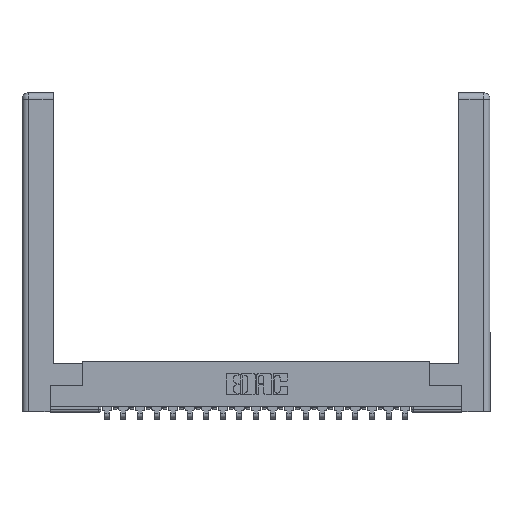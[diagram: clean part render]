
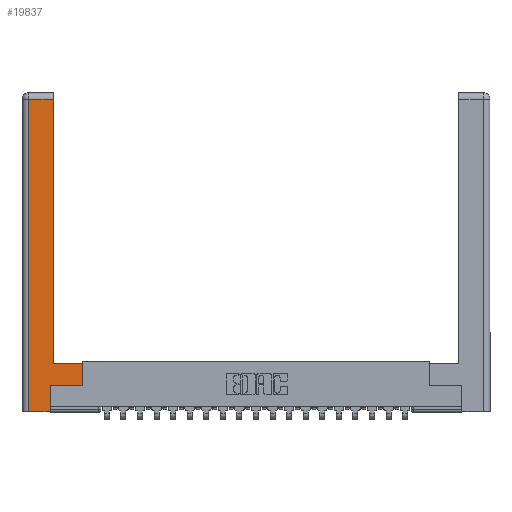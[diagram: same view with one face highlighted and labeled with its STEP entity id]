
A CAD part, top view. The second image highlights one B-rep face of the part: STEP entity #19837.
In plain terms, the highlighted planar face has unit normal (0, 0, 1).
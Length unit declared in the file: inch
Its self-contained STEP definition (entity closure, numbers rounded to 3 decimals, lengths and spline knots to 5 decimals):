
#886 = CARTESIAN_POINT ( 'NONE',  ( 0.565, 0.245, 0. ) ) ;
#1089 = DIRECTION ( 'NONE',  ( -1., 0., 0. ) ) ;
#1253 = ORIENTED_EDGE ( 'NONE', *, *, #11231, .T. ) ;
#1333 = VERTEX_POINT ( 'NONE', #20462 ) ;
#1446 = ORIENTED_EDGE ( 'NONE', *, *, #7583, .T. ) ;
#1805 = VECTOR ( 'NONE', #12024, 39.37008 ) ;
#2521 = FACE_OUTER_BOUND ( 'NONE', #11371, .T. ) ;
#2627 = EDGE_CURVE ( 'NONE', #5429, #12846, #7495, .T. ) ;
#4008 = ORIENTED_EDGE ( 'NONE', *, *, #13437, .T. ) ;
#4169 = CARTESIAN_POINT ( 'NONE',  ( 0.0615, 2.94, 0. ) ) ;
#4276 = VECTOR ( 'NONE', #11073, 39.37008 ) ;
#5429 = VERTEX_POINT ( 'NONE', #17028 ) ;
#5683 = EDGE_CURVE ( 'NONE', #12846, #7060, #19804, .T. ) ;
#6878 = VECTOR ( 'NONE', #13385, 39.37008 ) ;
#7042 = DIRECTION ( 'NONE',  ( 1., 0., 0. ) ) ;
#7044 = LINE ( 'NONE', #10290, #6878 ) ;
#7060 = VERTEX_POINT ( 'NONE', #20653 ) ;
#7122 = ORIENTED_EDGE ( 'NONE', *, *, #11388, .T. ) ;
#7495 = LINE ( 'NONE', #19582, #4276 ) ;
#7583 = EDGE_CURVE ( 'NONE', #1333, #17976, #12232, .T. ) ;
#7829 = ORIENTED_EDGE ( 'NONE', *, *, #5683, .T. ) ;
#8648 = AXIS2_PLACEMENT_3D ( 'NONE', #9257, #16247, #1089 ) ;
#9257 = CARTESIAN_POINT ( 'NONE',  ( 0., 0., 0. ) ) ;
#9922 = CARTESIAN_POINT ( 'NONE',  ( 0.565, 0.45, 0. ) ) ;
#9933 = CARTESIAN_POINT ( 'NONE',  ( 0.295, 0.45, 0. ) ) ;
#10170 = VERTEX_POINT ( 'NONE', #4169 ) ;
#10262 = VECTOR ( 'NONE', #16304, 39.37008 ) ;
#10290 = CARTESIAN_POINT ( 'NONE',  ( 0.0615, 0., 0. ) ) ;
#11041 = VERTEX_POINT ( 'NONE', #886 ) ;
#11073 = DIRECTION ( 'NONE',  ( 1., 0., 0. ) ) ;
#11139 = CARTESIAN_POINT ( 'NONE',  ( 0.265, 0., 0. ) ) ;
#11231 = EDGE_CURVE ( 'NONE', #11041, #15407, #16158, .T. ) ;
#11371 = EDGE_LOOP ( 'NONE', ( #1446, #18604, #7122, #17753, #7829, #4008, #1253, #19851 ) ) ;
#11388 = EDGE_CURVE ( 'NONE', #10170, #5429, #7044, .T. ) ;
#12024 = DIRECTION ( 'NONE',  ( 0., 1., 0. ) ) ;
#12232 = LINE ( 'NONE', #13456, #1805 ) ;
#12393 = CARTESIAN_POINT ( 'NONE',  ( 0.565, 0.245, 0. ) ) ;
#12846 = VERTEX_POINT ( 'NONE', #11139 ) ;
#12914 = DIRECTION ( 'NONE',  ( -1., 0., 0. ) ) ;
#13172 = DIRECTION ( 'NONE',  ( 0., 1., 0. ) ) ;
#13239 = LINE ( 'NONE', #9933, #17626 ) ;
#13385 = DIRECTION ( 'NONE',  ( 0., -1., 0. ) ) ;
#13437 = EDGE_CURVE ( 'NONE', #7060, #11041, #17353, .T. ) ;
#13456 = CARTESIAN_POINT ( 'NONE',  ( 0.295, 3., 0. ) ) ;
#14290 = CARTESIAN_POINT ( 'NONE',  ( 0.0615, 2.94, 0. ) ) ;
#14523 = LINE ( 'NONE', #14290, #10262 ) ;
#14919 = DIRECTION ( 'NONE',  ( 0., 1., 0. ) ) ;
#15016 = CARTESIAN_POINT ( 'NONE',  ( 0.265, 0.245, 0. ) ) ;
#15407 = VERTEX_POINT ( 'NONE', #9922 ) ;
#15787 = VECTOR ( 'NONE', #7042, 39.37008 ) ;
#15906 = PLANE ( 'NONE',  #8648 ) ;
#16117 = CARTESIAN_POINT ( 'NONE',  ( 0.295, 2.94, 0. ) ) ;
#16158 = LINE ( 'NONE', #21688, #21038 ) ;
#16247 = DIRECTION ( 'NONE',  ( 0., 0., -1. ) ) ;
#16304 = DIRECTION ( 'NONE',  ( -1., 0., 0. ) ) ;
#17028 = CARTESIAN_POINT ( 'NONE',  ( 0.0615, 0., 0. ) ) ;
#17353 = LINE ( 'NONE', #12393, #15787 ) ;
#17593 = EDGE_CURVE ( 'NONE', #17976, #10170, #14523, .T. ) ;
#17626 = VECTOR ( 'NONE', #12914, 39.37008 ) ;
#17675 = VECTOR ( 'NONE', #14919, 39.37008 ) ;
#17753 = ORIENTED_EDGE ( 'NONE', *, *, #2627, .T. ) ;
#17976 = VERTEX_POINT ( 'NONE', #16117 ) ;
#18079 = EDGE_CURVE ( 'NONE', #15407, #1333, #13239, .T. ) ;
#18604 = ORIENTED_EDGE ( 'NONE', *, *, #17593, .T. ) ;
#19582 = CARTESIAN_POINT ( 'NONE',  ( 0.265, 0., 0. ) ) ;
#19804 = LINE ( 'NONE', #15016, #17675 ) ;
#19837 = ADVANCED_FACE ( 'NONE', ( #2521 ), #15906, .F. ) ;
#19851 = ORIENTED_EDGE ( 'NONE', *, *, #18079, .T. ) ;
#20462 = CARTESIAN_POINT ( 'NONE',  ( 0.295, 0.45, 0. ) ) ;
#20653 = CARTESIAN_POINT ( 'NONE',  ( 0.265, 0.245, 0. ) ) ;
#21038 = VECTOR ( 'NONE', #13172, 39.37008 ) ;
#21688 = CARTESIAN_POINT ( 'NONE',  ( 0.565, 0.45, 0. ) ) ;
